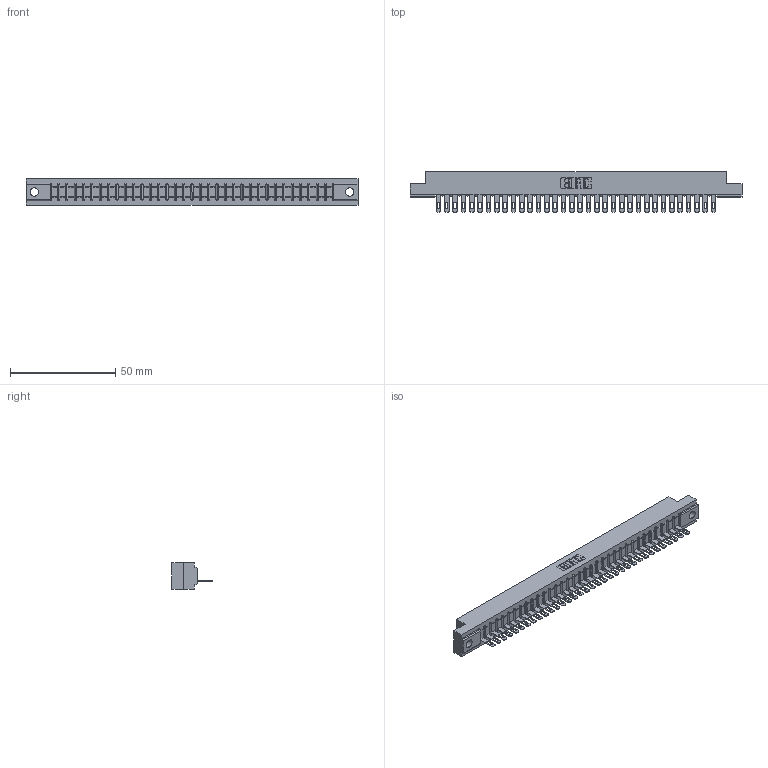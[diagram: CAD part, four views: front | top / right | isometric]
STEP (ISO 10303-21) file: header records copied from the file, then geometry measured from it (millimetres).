
FILE_DESCRIPTION (( 'STEP AP203' ), '1' );
FILE_NAME ('357-034-405-104.STEP', '2020-10-02T08:56:51', ( '' ), ( '' ), 'SwSTEP 2.0', 'SolidWorks 2020', '' );
FILE_SCHEMA (( 'CONFIG_CONTROL_DESIGN' ));
Length unit declared in the file: inch
Products named in the file (3): 307-290-001_505; 357-034-405-104; 307 Part_.156 Dia Mounting Holes
Assembly tree (35 placements, depth 2):
  357-034-405-104
    307 Part_.156 Dia Mounting Holes
    307-290-001_505  x34
Bounding box: 157.73 x 19.18 x 12.7 mm (x, y, z)
Volume: 16269.3 mm3; surface area: 17239.7 mm2
Topology: 35 solids, 35 shells, 2071 faces, 5867 edges, 3770 vertices
Faces by surface type: plane 1308, cylinder 693, sphere 70
Entity records: 30526 total; most frequent: CARTESIAN_POINT 5142, ORIENTED_EDGE 5126, DIRECTION 4999, EDGE_CURVE 2563, VECTOR 1969, LINE 1969, VERTEX_POINT 1658, AXIS2_PLACEMENT_3D 1515
